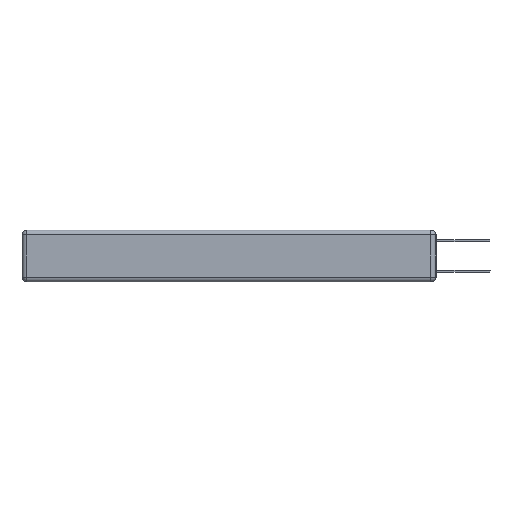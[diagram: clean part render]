
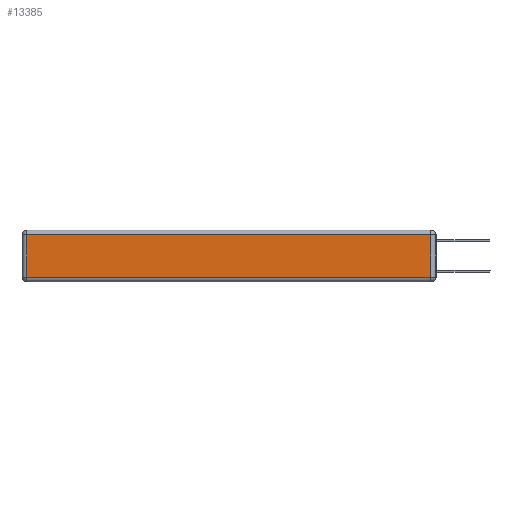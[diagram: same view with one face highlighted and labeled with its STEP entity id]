
A CAD part, left-side view. The second image highlights one B-rep face of the part: STEP entity #13385.
In plain terms, the highlighted planar face has unit normal (-1, 0, 0).
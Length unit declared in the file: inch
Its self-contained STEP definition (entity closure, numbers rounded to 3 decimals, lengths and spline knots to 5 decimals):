
#411 = CARTESIAN_POINT ( 'NONE',  ( 0., 2.75, -0.03 ) ) ;
#1534 = VECTOR ( 'NONE', #6845, 39.37008 ) ;
#2675 = CARTESIAN_POINT ( 'NONE',  ( 0., 0., -0.313 ) ) ;
#3876 = DIRECTION ( 'NONE',  ( 0., -1., 0. ) ) ;
#4679 = FACE_OUTER_BOUND ( 'NONE', #12589, .T. ) ;
#4853 = VECTOR ( 'NONE', #5010, 39.37008 ) ;
#5010 = DIRECTION ( 'NONE',  ( 0., 1., 0. ) ) ;
#5252 = VERTEX_POINT ( 'NONE', #8985 ) ;
#5751 = EDGE_CURVE ( 'NONE', #6438, #8303, #5893, .T. ) ;
#5799 = DIRECTION ( 'NONE',  ( -1., 0., 0. ) ) ;
#5893 = LINE ( 'NONE', #11345, #14338 ) ;
#6438 = VERTEX_POINT ( 'NONE', #11772 ) ;
#6588 = CARTESIAN_POINT ( 'NONE',  ( 0., 0.03, -0.03 ) ) ;
#6759 = VERTEX_POINT ( 'NONE', #12963 ) ;
#6845 = DIRECTION ( 'NONE',  ( 0., 0., -1. ) ) ;
#6855 = ORIENTED_EDGE ( 'NONE', *, *, #13431, .T. ) ;
#6909 = CARTESIAN_POINT ( 'NONE',  ( 0., 2.72, -0.343 ) ) ;
#7911 = DIRECTION ( 'NONE',  ( 0., 0., 1. ) ) ;
#8303 = VERTEX_POINT ( 'NONE', #6588 ) ;
#8913 = ORIENTED_EDGE ( 'NONE', *, *, #12628, .T. ) ;
#8985 = CARTESIAN_POINT ( 'NONE',  ( 0., 2.72, -0.313 ) ) ;
#9019 = DIRECTION ( 'NONE',  ( 0., 0., 1. ) ) ;
#9660 = VECTOR ( 'NONE', #3876, 39.37008 ) ;
#9875 = ORIENTED_EDGE ( 'NONE', *, *, #5751, .T. ) ;
#10832 = LINE ( 'NONE', #2675, #9660 ) ;
#10916 = LINE ( 'NONE', #411, #4853 ) ;
#11248 = CARTESIAN_POINT ( 'NONE',  ( 0., 0., -0.343 ) ) ;
#11258 = EDGE_CURVE ( 'NONE', #8303, #6759, #10916, .T. ) ;
#11345 = CARTESIAN_POINT ( 'NONE',  ( 0., 0.03, -0.343 ) ) ;
#11772 = CARTESIAN_POINT ( 'NONE',  ( 0., 0.03, -0.313 ) ) ;
#11870 = ORIENTED_EDGE ( 'NONE', *, *, #11258, .T. ) ;
#12589 = EDGE_LOOP ( 'NONE', ( #8913, #9875, #11870, #6855 ) ) ;
#12628 = EDGE_CURVE ( 'NONE', #5252, #6438, #10832, .T. ) ;
#12748 = PLANE ( 'NONE',  #13730 ) ;
#12963 = CARTESIAN_POINT ( 'NONE',  ( 0., 2.72, -0.03 ) ) ;
#13385 = ADVANCED_FACE ( 'NONE', ( #4679 ), #12748, .T. ) ;
#13431 = EDGE_CURVE ( 'NONE', #6759, #5252, #14779, .T. ) ;
#13730 = AXIS2_PLACEMENT_3D ( 'NONE', #11248, #5799, #9019 ) ;
#14338 = VECTOR ( 'NONE', #7911, 39.37008 ) ;
#14779 = LINE ( 'NONE', #6909, #1534 ) ;
